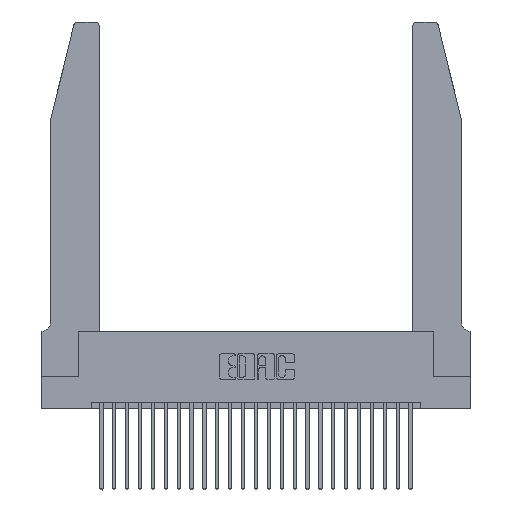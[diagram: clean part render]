
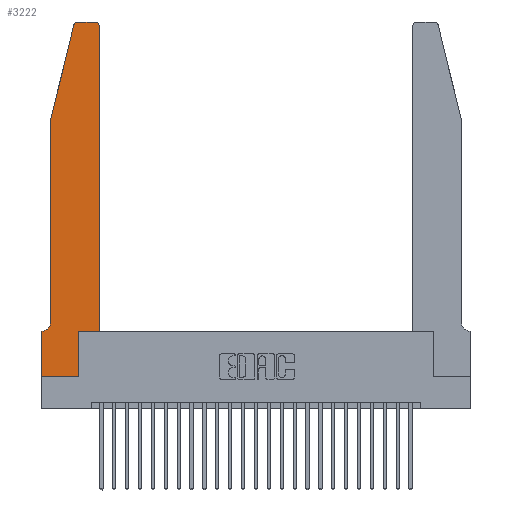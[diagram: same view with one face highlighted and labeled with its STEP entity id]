
A CAD part, top view. The second image highlights one B-rep face of the part: STEP entity #3222.
In plain terms, the highlighted planar face has unit normal (0, 0, 1).
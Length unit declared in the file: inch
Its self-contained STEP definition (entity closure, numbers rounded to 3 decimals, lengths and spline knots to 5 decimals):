
#126 = AXIS2_PLACEMENT_3D ( 'NONE', #14885, #8976, #21142 ) ;
#148 = ORIENTED_EDGE ( 'NONE', *, *, #21308, .T. ) ;
#654 = CARTESIAN_POINT ( 'NONE',  ( 0.2605, 2.75, 0.37 ) ) ;
#826 = VECTOR ( 'NONE', #16883, 39.37008 ) ;
#846 = CARTESIAN_POINT ( 'NONE',  ( 0.25487, 2.72718, 0.37 ) ) ;
#966 = EDGE_LOOP ( 'NONE', ( #20660, #15901, #3421, #13324, #22754, #5107, #16112, #148, #14697, #23768, #22843, #26315 ) ) ;
#1956 = LINE ( 'NONE', #23751, #20908 ) ;
#2089 = CARTESIAN_POINT ( 'NONE',  ( 0.2865, 0.35, 0.37 ) ) ;
#2628 = DIRECTION ( 'NONE',  ( 0., -1., 0. ) ) ;
#2654 = DIRECTION ( 'NONE',  ( 1., 0., 0. ) ) ;
#3155 = VERTEX_POINT ( 'NONE', #12554 ) ;
#3222 = ADVANCED_FACE ( 'NONE', ( #25588 ), #21330, .T. ) ;
#3234 = CARTESIAN_POINT ( 'NONE',  ( 0.4205, 2.75, 0.37 ) ) ;
#3263 = LINE ( 'NONE', #14413, #6442 ) ;
#3421 = ORIENTED_EDGE ( 'NONE', *, *, #6130, .T. ) ;
#3606 = DIRECTION ( 'NONE',  ( 1., 0., 0. ) ) ;
#3702 = VERTEX_POINT ( 'NONE', #6330 ) ;
#3757 = VERTEX_POINT ( 'NONE', #2089 ) ;
#3895 = DIRECTION ( 'NONE',  ( 0., 0., 1. ) ) ;
#4927 = CARTESIAN_POINT ( 'NONE',  ( 0.0055, 0.42, 0.37 ) ) ;
#5107 = ORIENTED_EDGE ( 'NONE', *, *, #11292, .T. ) ;
#5809 = LINE ( 'NONE', #12435, #18336 ) ;
#5942 = LINE ( 'NONE', #22732, #6908 ) ;
#6130 = EDGE_CURVE ( 'NONE', #12815, #11650, #10760, .T. ) ;
#6330 = CARTESIAN_POINT ( 'NONE',  ( 0.2865, 0., 0.37 ) ) ;
#6442 = VECTOR ( 'NONE', #8492, 39.37008 ) ;
#6549 = CARTESIAN_POINT ( 'NONE',  ( 0.284, 2.72, 0.37 ) ) ;
#6702 = EDGE_CURVE ( 'NONE', #10838, #19462, #17206, .T. ) ;
#6908 = VECTOR ( 'NONE', #10304, 39.37008 ) ;
#7083 = CARTESIAN_POINT ( 'NONE',  ( 0.4505, 2.72, 0.37 ) ) ;
#8492 = DIRECTION ( 'NONE',  ( -1., 0., 0. ) ) ;
#8976 = DIRECTION ( 'NONE',  ( 0., 0., 1. ) ) ;
#8980 = DIRECTION ( 'NONE',  ( 0., 0., 1. ) ) ;
#9019 = DIRECTION ( 'NONE',  ( 0., 0., -1. ) ) ;
#9155 = VERTEX_POINT ( 'NONE', #22229 ) ;
#9271 = DIRECTION ( 'NONE',  ( -1., 0., 0. ) ) ;
#10304 = DIRECTION ( 'NONE',  ( 0., 1., 0. ) ) ;
#10760 = LINE ( 'NONE', #23110, #22435 ) ;
#10838 = VERTEX_POINT ( 'NONE', #13082 ) ;
#11102 = DIRECTION ( 'NONE',  ( 1., 0., 0. ) ) ;
#11292 = EDGE_CURVE ( 'NONE', #25584, #19840, #3263, .T. ) ;
#11337 = EDGE_CURVE ( 'NONE', #11650, #9155, #5809, .T. ) ;
#11650 = VERTEX_POINT ( 'NONE', #24001 ) ;
#12265 = CARTESIAN_POINT ( 'NONE',  ( 0., 0., 0.37 ) ) ;
#12435 = CARTESIAN_POINT ( 'NONE',  ( 0.0755, 2., 0.37 ) ) ;
#12554 = CARTESIAN_POINT ( 'NONE',  ( 0.284, 2.75, 0.37 ) ) ;
#12815 = VERTEX_POINT ( 'NONE', #846 ) ;
#12858 = DIRECTION ( 'NONE',  ( -0.239, -0.971, 0. ) ) ;
#13005 = VECTOR ( 'NONE', #11102, 39.37008 ) ;
#13082 = CARTESIAN_POINT ( 'NONE',  ( 0.4505, 0.35, 0.37 ) ) ;
#13324 = ORIENTED_EDGE ( 'NONE', *, *, #11337, .T. ) ;
#13547 = CIRCLE ( 'NONE', #126, 0.03 ) ;
#13868 = CIRCLE ( 'NONE', #16827, 0.03 ) ;
#14413 = CARTESIAN_POINT ( 'NONE',  ( 0.0755, 0.35, 0.37 ) ) ;
#14681 = CARTESIAN_POINT ( 'NONE',  ( 0., 0.35, 0.37 ) ) ;
#14697 = ORIENTED_EDGE ( 'NONE', *, *, #16281, .T. ) ;
#14781 = CARTESIAN_POINT ( 'NONE',  ( 0.4505, 0.35, 0.37 ) ) ;
#14885 = CARTESIAN_POINT ( 'NONE',  ( 0.4205, 2.72, 0.37 ) ) ;
#15054 = EDGE_CURVE ( 'NONE', #17659, #3155, #16545, .T. ) ;
#15591 = DIRECTION ( 'NONE',  ( 0., -1., 0. ) ) ;
#15901 = ORIENTED_EDGE ( 'NONE', *, *, #18681, .T. ) ;
#16112 = ORIENTED_EDGE ( 'NONE', *, *, #21265, .T. ) ;
#16281 = EDGE_CURVE ( 'NONE', #3702, #3757, #5942, .T. ) ;
#16545 = LINE ( 'NONE', #654, #18500 ) ;
#16827 = AXIS2_PLACEMENT_3D ( 'NONE', #6549, #3895, #22962 ) ;
#16883 = DIRECTION ( 'NONE',  ( 0., 1., 0. ) ) ;
#17196 = CIRCLE ( 'NONE', #25830, 0.07 ) ;
#17206 = LINE ( 'NONE', #14781, #826 ) ;
#17511 = EDGE_CURVE ( 'NONE', #9155, #25584, #17196, .T. ) ;
#17659 = VERTEX_POINT ( 'NONE', #3234 ) ;
#17664 = LINE ( 'NONE', #18036, #18650 ) ;
#18036 = CARTESIAN_POINT ( 'NONE',  ( 0., 0., 0.37 ) ) ;
#18336 = VECTOR ( 'NONE', #2628, 39.37008 ) ;
#18500 = VECTOR ( 'NONE', #21318, 39.37008 ) ;
#18650 = VECTOR ( 'NONE', #3606, 39.37008 ) ;
#18681 = EDGE_CURVE ( 'NONE', #3155, #12815, #13868, .T. ) ;
#18796 = EDGE_CURVE ( 'NONE', #19462, #17659, #13547, .T. ) ;
#19462 = VERTEX_POINT ( 'NONE', #7083 ) ;
#19485 = LINE ( 'NONE', #25763, #13005 ) ;
#19840 = VERTEX_POINT ( 'NONE', #14681 ) ;
#20660 = ORIENTED_EDGE ( 'NONE', *, *, #15054, .T. ) ;
#20908 = VECTOR ( 'NONE', #15591, 39.37008 ) ;
#20920 = CARTESIAN_POINT ( 'NONE',  ( 0.0055, 0.35, 0.37 ) ) ;
#21142 = DIRECTION ( 'NONE',  ( 1., 0., 0. ) ) ;
#21265 = EDGE_CURVE ( 'NONE', #19840, #22966, #1956, .T. ) ;
#21308 = EDGE_CURVE ( 'NONE', #22966, #3702, #17664, .T. ) ;
#21318 = DIRECTION ( 'NONE',  ( -1., 0., 0. ) ) ;
#21330 = PLANE ( 'NONE',  #24416 ) ;
#22229 = CARTESIAN_POINT ( 'NONE',  ( 0.0755, 0.42, 0.37 ) ) ;
#22435 = VECTOR ( 'NONE', #12858, 39.37008 ) ;
#22732 = CARTESIAN_POINT ( 'NONE',  ( 0.2865, 0.35, 0.37 ) ) ;
#22754 = ORIENTED_EDGE ( 'NONE', *, *, #17511, .T. ) ;
#22843 = ORIENTED_EDGE ( 'NONE', *, *, #6702, .T. ) ;
#22962 = DIRECTION ( 'NONE',  ( 1., 0., 0. ) ) ;
#22966 = VERTEX_POINT ( 'NONE', #12265 ) ;
#23110 = CARTESIAN_POINT ( 'NONE',  ( 0.0755, 2., 0.37 ) ) ;
#23751 = CARTESIAN_POINT ( 'NONE',  ( 0., 0., 0.37 ) ) ;
#23768 = ORIENTED_EDGE ( 'NONE', *, *, #25249, .T. ) ;
#24001 = CARTESIAN_POINT ( 'NONE',  ( 0.0755, 2., 0.37 ) ) ;
#24416 = AXIS2_PLACEMENT_3D ( 'NONE', #25333, #8980, #2654 ) ;
#25249 = EDGE_CURVE ( 'NONE', #3757, #10838, #19485, .T. ) ;
#25333 = CARTESIAN_POINT ( 'NONE',  ( 0., 0.35, 0.37 ) ) ;
#25584 = VERTEX_POINT ( 'NONE', #20920 ) ;
#25588 = FACE_OUTER_BOUND ( 'NONE', #966, .T. ) ;
#25763 = CARTESIAN_POINT ( 'NONE',  ( 0.4505, 0.35, 0.37 ) ) ;
#25830 = AXIS2_PLACEMENT_3D ( 'NONE', #4927, #9019, #9271 ) ;
#26315 = ORIENTED_EDGE ( 'NONE', *, *, #18796, .T. ) ;
